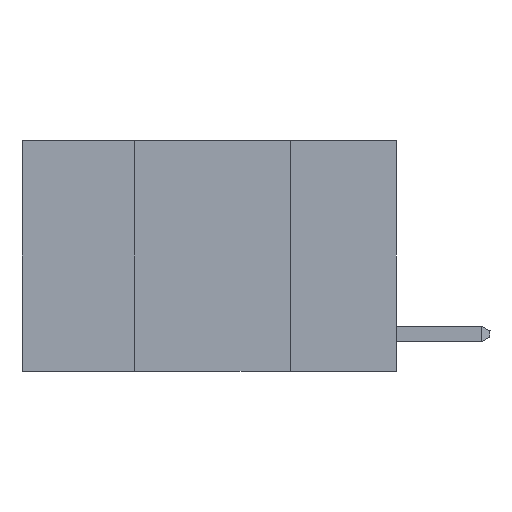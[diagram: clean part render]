
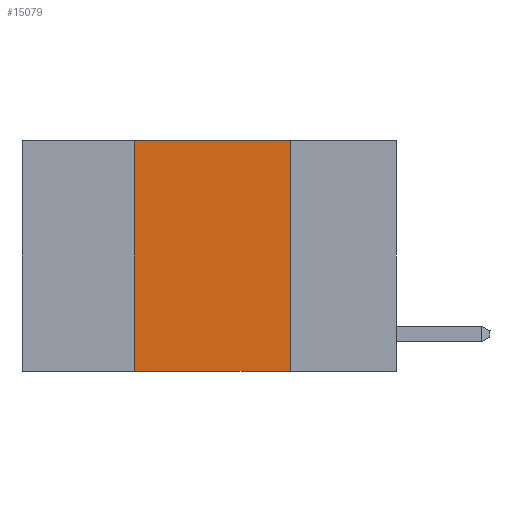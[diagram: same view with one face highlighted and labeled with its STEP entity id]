
A CAD part, left-side view. The second image highlights one B-rep face of the part: STEP entity #15079.
In plain terms, the highlighted planar face has unit normal (-1, 0, 0).
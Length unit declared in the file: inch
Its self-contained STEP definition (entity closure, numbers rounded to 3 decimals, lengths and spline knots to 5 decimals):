
#1045 = CARTESIAN_POINT ( 'NONE',  ( 0., 0.17, 0. ) ) ;
#2109 = ORIENTED_EDGE ( 'NONE', *, *, #13021, .F. ) ;
#3166 = ORIENTED_EDGE ( 'NONE', *, *, #7767, .T. ) ;
#3956 = EDGE_LOOP ( 'NONE', ( #2109, #8710, #10806, #3166 ) ) ;
#5333 = FACE_OUTER_BOUND ( 'NONE', #3956, .T. ) ;
#5507 = CARTESIAN_POINT ( 'NONE',  ( 0., 0.6, 0. ) ) ;
#5610 = CARTESIAN_POINT ( 'NONE',  ( 0., 0.42, 0. ) ) ;
#6498 = VERTEX_POINT ( 'NONE', #18502 ) ;
#6634 = DIRECTION ( 'NONE',  ( 1., 0., 0. ) ) ;
#6777 = DIRECTION ( 'NONE',  ( 0., 0., 1. ) ) ;
#6823 = VECTOR ( 'NONE', #6777, 39.37008 ) ;
#7115 = DIRECTION ( 'NONE',  ( 0., -1., 0. ) ) ;
#7767 = EDGE_CURVE ( 'NONE', #11413, #6498, #18694, .T. ) ;
#8710 = ORIENTED_EDGE ( 'NONE', *, *, #9254, .F. ) ;
#9254 = EDGE_CURVE ( 'NONE', #10546, #13614, #13058, .T. ) ;
#10546 = VERTEX_POINT ( 'NONE', #5610 ) ;
#10568 = CARTESIAN_POINT ( 'NONE',  ( 0., 0.6, -0.37 ) ) ;
#10806 = ORIENTED_EDGE ( 'NONE', *, *, #12651, .F. ) ;
#11127 = CARTESIAN_POINT ( 'NONE',  ( 0., 0.42, 0. ) ) ;
#11413 = VERTEX_POINT ( 'NONE', #16197 ) ;
#11609 = AXIS2_PLACEMENT_3D ( 'NONE', #17257, #6634, #19038 ) ;
#12651 = EDGE_CURVE ( 'NONE', #11413, #10546, #18691, .T. ) ;
#12777 = PLANE ( 'NONE',  #11609 ) ;
#12983 = LINE ( 'NONE', #1045, #13447 ) ;
#13021 = EDGE_CURVE ( 'NONE', #13614, #6498, #12983, .T. ) ;
#13058 = LINE ( 'NONE', #5507, #13526 ) ;
#13447 = VECTOR ( 'NONE', #14476, 39.37008 ) ;
#13526 = VECTOR ( 'NONE', #7115, 39.37008 ) ;
#13614 = VERTEX_POINT ( 'NONE', #18718 ) ;
#14476 = DIRECTION ( 'NONE',  ( 0., 0., -1. ) ) ;
#15079 = ADVANCED_FACE ( 'NONE', ( #5333 ), #12777, .F. ) ;
#16197 = CARTESIAN_POINT ( 'NONE',  ( 0., 0.42, -0.37 ) ) ;
#17257 = CARTESIAN_POINT ( 'NONE',  ( 0., 0.6, 0. ) ) ;
#17373 = VECTOR ( 'NONE', #18237, 39.37008 ) ;
#18237 = DIRECTION ( 'NONE',  ( 0., -1., 0. ) ) ;
#18502 = CARTESIAN_POINT ( 'NONE',  ( 0., 0.17, -0.37 ) ) ;
#18691 = LINE ( 'NONE', #11127, #6823 ) ;
#18694 = LINE ( 'NONE', #10568, #17373 ) ;
#18718 = CARTESIAN_POINT ( 'NONE',  ( 0., 0.17, 0. ) ) ;
#19038 = DIRECTION ( 'NONE',  ( 0., 0., -1. ) ) ;
